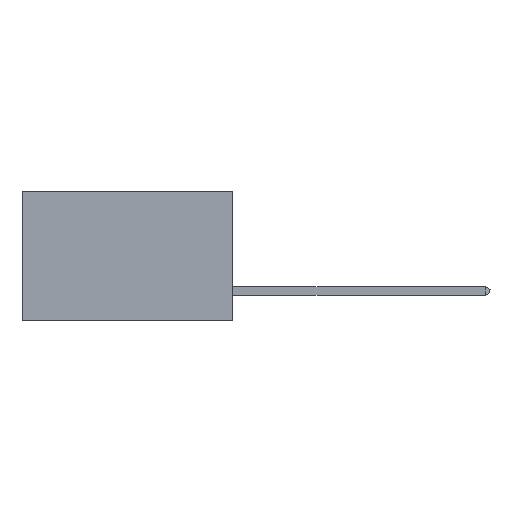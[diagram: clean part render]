
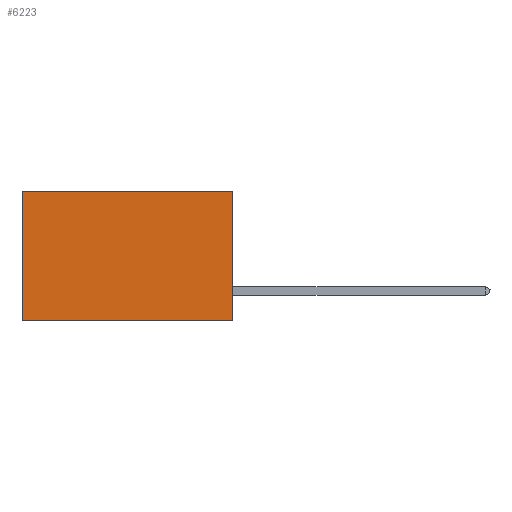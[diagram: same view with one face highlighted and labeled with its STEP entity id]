
A CAD part, left-side view. The second image highlights one B-rep face of the part: STEP entity #6223.
In plain terms, the highlighted planar face has unit normal (-1, 0, 0).
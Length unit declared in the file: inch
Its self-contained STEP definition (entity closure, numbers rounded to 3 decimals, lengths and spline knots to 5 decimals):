
#154 = FACE_OUTER_BOUND ( 'NONE', #12198, .T. ) ;
#339 = LINE ( 'NONE', #10496, #3429 ) ;
#448 = PLANE ( 'NONE',  #4294 ) ;
#1514 = VERTEX_POINT ( 'NONE', #12469 ) ;
#2572 = CARTESIAN_POINT ( 'NONE',  ( 0.2875, 0., 0. ) ) ;
#2610 = LINE ( 'NONE', #5914, #13112 ) ;
#3090 = CARTESIAN_POINT ( 'NONE',  ( 0.2875, 0.6, 0. ) ) ;
#3429 = VECTOR ( 'NONE', #4285, 39.37008 ) ;
#3684 = ORIENTED_EDGE ( 'NONE', *, *, #5241, .F. ) ;
#3804 = LINE ( 'NONE', #2572, #4774 ) ;
#4260 = VERTEX_POINT ( 'NONE', #10629 ) ;
#4285 = DIRECTION ( 'NONE',  ( 0., 0., -1. ) ) ;
#4294 = AXIS2_PLACEMENT_3D ( 'NONE', #12818, #9890, #7711 ) ;
#4774 = VECTOR ( 'NONE', #12108, 39.37008 ) ;
#4959 = ORIENTED_EDGE ( 'NONE', *, *, #10840, .T. ) ;
#5170 = VECTOR ( 'NONE', #12997, 39.37008 ) ;
#5180 = VERTEX_POINT ( 'NONE', #5197 ) ;
#5197 = CARTESIAN_POINT ( 'NONE',  ( 0.2875, 0., 0. ) ) ;
#5241 = EDGE_CURVE ( 'NONE', #5180, #4260, #339, .T. ) ;
#5701 = VERTEX_POINT ( 'NONE', #3090 ) ;
#5914 = CARTESIAN_POINT ( 'NONE',  ( 0.2875, 0.6, 0. ) ) ;
#6208 = EDGE_CURVE ( 'NONE', #4260, #1514, #7905, .T. ) ;
#6223 = ADVANCED_FACE ( 'NONE', ( #154 ), #448, .F. ) ;
#6873 = ORIENTED_EDGE ( 'NONE', *, *, #8854, .T. ) ;
#7711 = DIRECTION ( 'NONE',  ( 0., 0., -1. ) ) ;
#7905 = LINE ( 'NONE', #12863, #5170 ) ;
#8854 = EDGE_CURVE ( 'NONE', #5701, #1514, #2610, .T. ) ;
#9890 = DIRECTION ( 'NONE',  ( 1., 0., 0. ) ) ;
#10496 = CARTESIAN_POINT ( 'NONE',  ( 0.2875, 0., 0. ) ) ;
#10629 = CARTESIAN_POINT ( 'NONE',  ( 0.2875, 0., -0.37 ) ) ;
#10840 = EDGE_CURVE ( 'NONE', #5180, #5701, #3804, .T. ) ;
#11243 = ORIENTED_EDGE ( 'NONE', *, *, #6208, .F. ) ;
#12108 = DIRECTION ( 'NONE',  ( 0., 1., 0. ) ) ;
#12198 = EDGE_LOOP ( 'NONE', ( #6873, #11243, #3684, #4959 ) ) ;
#12469 = CARTESIAN_POINT ( 'NONE',  ( 0.2875, 0.6, -0.37 ) ) ;
#12818 = CARTESIAN_POINT ( 'NONE',  ( 0.2875, 0., 0. ) ) ;
#12863 = CARTESIAN_POINT ( 'NONE',  ( 0.2875, 0., -0.37 ) ) ;
#12997 = DIRECTION ( 'NONE',  ( 0., 1., 0. ) ) ;
#13112 = VECTOR ( 'NONE', #13241, 39.37008 ) ;
#13241 = DIRECTION ( 'NONE',  ( 0., 0., -1. ) ) ;
